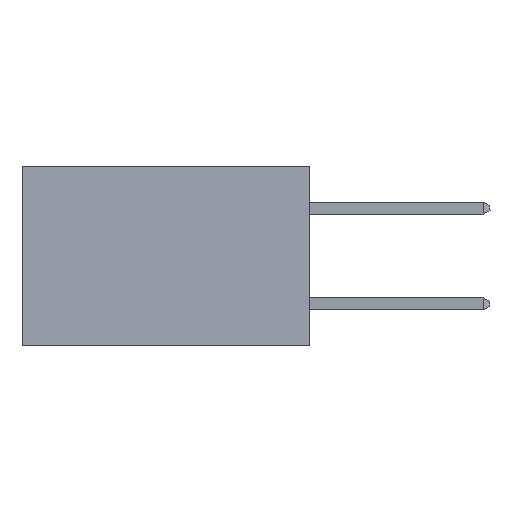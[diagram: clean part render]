
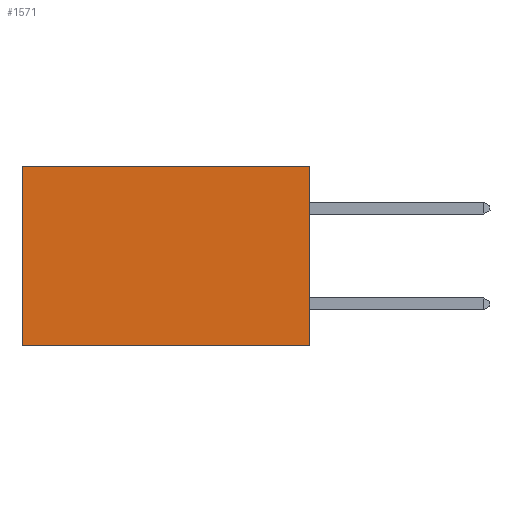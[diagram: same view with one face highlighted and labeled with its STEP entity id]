
A CAD part, left-side view. The second image highlights one B-rep face of the part: STEP entity #1571.
In plain terms, the highlighted planar face has unit normal (-1, 0, 0).
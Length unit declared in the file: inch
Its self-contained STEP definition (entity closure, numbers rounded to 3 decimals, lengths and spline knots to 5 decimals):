
#247 = VECTOR ( 'NONE', #789, 39.37008 ) ;
#789 = DIRECTION ( 'NONE',  ( 0., 0., -1. ) ) ;
#944 = ORIENTED_EDGE ( 'NONE', *, *, #6281, .F. ) ;
#1100 = EDGE_CURVE ( 'NONE', #2823, #2765, #2419, .T. ) ;
#1190 = ORIENTED_EDGE ( 'NONE', *, *, #1100, .F. ) ;
#1291 = LINE ( 'NONE', #4416, #1996 ) ;
#1571 = ADVANCED_FACE ( 'NONE', ( #7116 ), #4869, .F. ) ;
#1996 = VECTOR ( 'NONE', #6903, 39.37008 ) ;
#1999 = EDGE_CURVE ( 'NONE', #3165, #2765, #7503, .T. ) ;
#2220 = VERTEX_POINT ( 'NONE', #3468 ) ;
#2419 = LINE ( 'NONE', #6200, #4320 ) ;
#2765 = VERTEX_POINT ( 'NONE', #7207 ) ;
#2823 = VERTEX_POINT ( 'NONE', #6493 ) ;
#2994 = DIRECTION ( 'NONE',  ( 0., 0., -1. ) ) ;
#3053 = EDGE_CURVE ( 'NONE', #2220, #3165, #1291, .T. ) ;
#3160 = DIRECTION ( 'NONE',  ( 0., 1., 0. ) ) ;
#3165 = VERTEX_POINT ( 'NONE', #4524 ) ;
#3468 = CARTESIAN_POINT ( 'NONE',  ( 0.2875, 0., 0. ) ) ;
#3829 = LINE ( 'NONE', #5848, #247 ) ;
#4242 = CARTESIAN_POINT ( 'NONE',  ( 0.2875, 0., -0.375 ) ) ;
#4320 = VECTOR ( 'NONE', #3160, 39.37008 ) ;
#4382 = AXIS2_PLACEMENT_3D ( 'NONE', #4242, #5511, #2994 ) ;
#4416 = CARTESIAN_POINT ( 'NONE',  ( 0.2875, 0., 0. ) ) ;
#4517 = CARTESIAN_POINT ( 'NONE',  ( 0.2875, 0.6, -0.375 ) ) ;
#4524 = CARTESIAN_POINT ( 'NONE',  ( 0.2875, 0.6, 0. ) ) ;
#4869 = PLANE ( 'NONE',  #4382 ) ;
#5511 = DIRECTION ( 'NONE',  ( 1., 0., 0. ) ) ;
#5848 = CARTESIAN_POINT ( 'NONE',  ( 0.2875, 0., -0.375 ) ) ;
#6200 = CARTESIAN_POINT ( 'NONE',  ( 0.2875, 0., -0.375 ) ) ;
#6281 = EDGE_CURVE ( 'NONE', #2220, #2823, #3829, .T. ) ;
#6493 = CARTESIAN_POINT ( 'NONE',  ( 0.2875, 0., -0.375 ) ) ;
#6741 = ORIENTED_EDGE ( 'NONE', *, *, #3053, .T. ) ;
#6776 = EDGE_LOOP ( 'NONE', ( #8227, #1190, #944, #6741 ) ) ;
#6903 = DIRECTION ( 'NONE',  ( 0., 1., 0. ) ) ;
#7111 = VECTOR ( 'NONE', #7787, 39.37008 ) ;
#7116 = FACE_OUTER_BOUND ( 'NONE', #6776, .T. ) ;
#7207 = CARTESIAN_POINT ( 'NONE',  ( 0.2875, 0.6, -0.375 ) ) ;
#7503 = LINE ( 'NONE', #4517, #7111 ) ;
#7787 = DIRECTION ( 'NONE',  ( 0., 0., -1. ) ) ;
#8227 = ORIENTED_EDGE ( 'NONE', *, *, #1999, .T. ) ;
